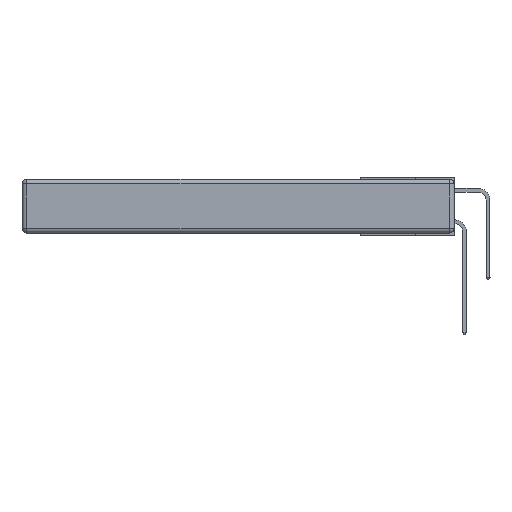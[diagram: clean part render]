
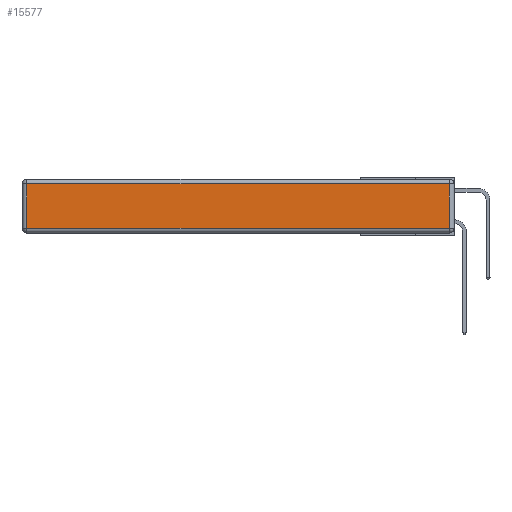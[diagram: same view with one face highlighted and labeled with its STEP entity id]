
A CAD part, left-side view. The second image highlights one B-rep face of the part: STEP entity #15577.
In plain terms, the highlighted planar face has unit normal (-1, 0, 0).
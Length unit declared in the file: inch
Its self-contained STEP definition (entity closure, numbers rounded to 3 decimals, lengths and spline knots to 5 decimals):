
#676 = DIRECTION ( 'NONE',  ( 0., 0., -1. ) ) ;
#916 = CARTESIAN_POINT ( 'NONE',  ( 0., 0.03, -0.313 ) ) ;
#1135 = DIRECTION ( 'NONE',  ( 0., 0., 1. ) ) ;
#2125 = VECTOR ( 'NONE', #22884, 39.37008 ) ;
#4347 = CARTESIAN_POINT ( 'NONE',  ( 0., 2.75, -0.03 ) ) ;
#5504 = ORIENTED_EDGE ( 'NONE', *, *, #30532, .T. ) ;
#6718 = FACE_OUTER_BOUND ( 'NONE', #15194, .T. ) ;
#7051 = ORIENTED_EDGE ( 'NONE', *, *, #10187, .T. ) ;
#9130 = DIRECTION ( 'NONE',  ( 0., 0., 1. ) ) ;
#10187 = EDGE_CURVE ( 'NONE', #27876, #11406, #31869, .T. ) ;
#10982 = LINE ( 'NONE', #32776, #18664 ) ;
#11406 = VERTEX_POINT ( 'NONE', #31494 ) ;
#13479 = ORIENTED_EDGE ( 'NONE', *, *, #23243, .T. ) ;
#14388 = LINE ( 'NONE', #34654, #25958 ) ;
#15194 = EDGE_LOOP ( 'NONE', ( #32016, #13479, #7051, #5504 ) ) ;
#15577 = ADVANCED_FACE ( 'NONE', ( #6718 ), #17943, .T. ) ;
#17439 = DIRECTION ( 'NONE',  ( -1., 0., 0. ) ) ;
#17477 = CARTESIAN_POINT ( 'NONE',  ( 0., 0.03, -0.343 ) ) ;
#17943 = PLANE ( 'NONE',  #23661 ) ;
#18123 = CARTESIAN_POINT ( 'NONE',  ( 0., 2.72, -0.313 ) ) ;
#18408 = DIRECTION ( 'NONE',  ( 0., -1., 0. ) ) ;
#18664 = VECTOR ( 'NONE', #676, 39.37008 ) ;
#20017 = VERTEX_POINT ( 'NONE', #18123 ) ;
#22884 = DIRECTION ( 'NONE',  ( 0., 1., 0. ) ) ;
#23243 = EDGE_CURVE ( 'NONE', #34927, #27876, #28480, .T. ) ;
#23405 = CARTESIAN_POINT ( 'NONE',  ( 0., 0., -0.343 ) ) ;
#23661 = AXIS2_PLACEMENT_3D ( 'NONE', #23405, #17439, #1135 ) ;
#24010 = CARTESIAN_POINT ( 'NONE',  ( 0., 0.03, -0.03 ) ) ;
#25958 = VECTOR ( 'NONE', #18408, 39.37008 ) ;
#27876 = VERTEX_POINT ( 'NONE', #24010 ) ;
#28480 = LINE ( 'NONE', #17477, #34811 ) ;
#30532 = EDGE_CURVE ( 'NONE', #11406, #20017, #10982, .T. ) ;
#31494 = CARTESIAN_POINT ( 'NONE',  ( 0., 2.72, -0.03 ) ) ;
#31869 = LINE ( 'NONE', #4347, #2125 ) ;
#32016 = ORIENTED_EDGE ( 'NONE', *, *, #32660, .T. ) ;
#32660 = EDGE_CURVE ( 'NONE', #20017, #34927, #14388, .T. ) ;
#32776 = CARTESIAN_POINT ( 'NONE',  ( 0., 2.72, -0.343 ) ) ;
#34654 = CARTESIAN_POINT ( 'NONE',  ( 0., 0., -0.313 ) ) ;
#34811 = VECTOR ( 'NONE', #9130, 39.37008 ) ;
#34927 = VERTEX_POINT ( 'NONE', #916 ) ;
